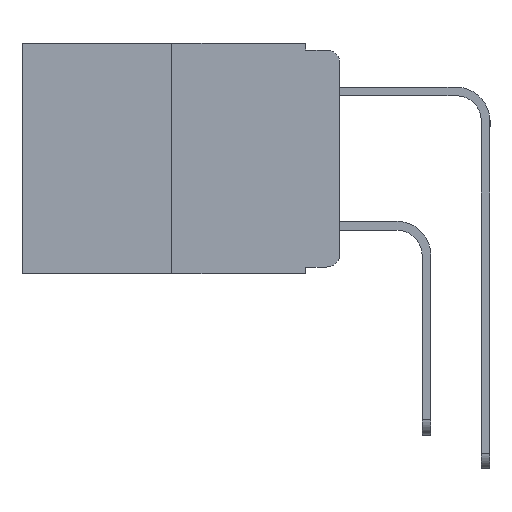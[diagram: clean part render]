
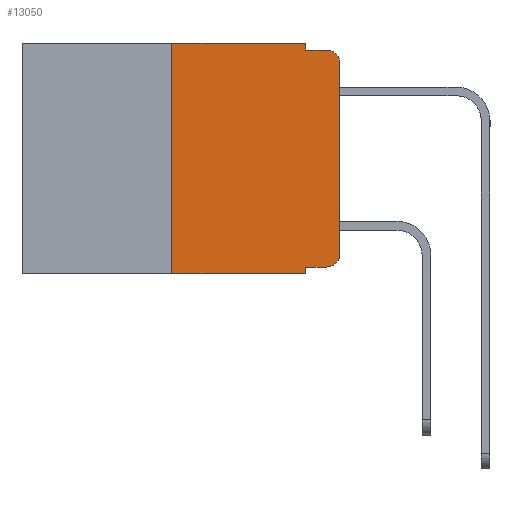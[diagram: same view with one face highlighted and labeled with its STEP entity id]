
A CAD part, left-side view. The second image highlights one B-rep face of the part: STEP entity #13050.
In plain terms, the highlighted planar face has unit normal (-1, 0, 0).
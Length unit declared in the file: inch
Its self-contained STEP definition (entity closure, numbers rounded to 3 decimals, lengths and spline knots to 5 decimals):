
#21 = CARTESIAN_POINT ( 'NONE',  ( 0., 0.051, -0.343 ) ) ;
#23 = CARTESIAN_POINT ( 'NONE',  ( 0., 0.02, -0.313 ) ) ;
#226 = EDGE_CURVE ( 'NONE', #5284, #3905, #3051, .T. ) ;
#235 = VECTOR ( 'NONE', #8747, 39.37008 ) ;
#519 = DIRECTION ( 'NONE',  ( 1., 0., 0. ) ) ;
#1103 = EDGE_CURVE ( 'NONE', #12461, #7772, #3863, .T. ) ;
#1113 = VERTEX_POINT ( 'NONE', #21 ) ;
#1264 = ORIENTED_EDGE ( 'NONE', *, *, #11909, .T. ) ;
#1349 = DIRECTION ( 'NONE',  ( 0., 0., -1. ) ) ;
#1474 = VERTEX_POINT ( 'NONE', #14182 ) ;
#1689 = ORIENTED_EDGE ( 'NONE', *, *, #14249, .F. ) ;
#1947 = EDGE_CURVE ( 'NONE', #7772, #6663, #12931, .T. ) ;
#2248 = CARTESIAN_POINT ( 'NONE',  ( 0., 0.051, 0. ) ) ;
#2265 = ORIENTED_EDGE ( 'NONE', *, *, #1947, .F. ) ;
#2275 = EDGE_LOOP ( 'NONE', ( #10076, #11959, #2265, #11504, #1689, #5946, #6763, #6268, #1264, #14040 ) ) ;
#2479 = CARTESIAN_POINT ( 'NONE',  ( 0., 0.473, -0.343 ) ) ;
#2789 = EDGE_CURVE ( 'NONE', #13586, #6663, #13840, .T. ) ;
#2926 = DIRECTION ( 'NONE',  ( -1., 0., 0. ) ) ;
#2942 = VERTEX_POINT ( 'NONE', #5293 ) ;
#2943 = VECTOR ( 'NONE', #12343, 39.37008 ) ;
#2957 = CARTESIAN_POINT ( 'NONE',  ( 0., 0.02, -0.03 ) ) ;
#3022 = CIRCLE ( 'NONE', #9111, 0.02 ) ;
#3051 = LINE ( 'NONE', #4029, #14140 ) ;
#3410 = CARTESIAN_POINT ( 'NONE',  ( 0., 0.02, -0.01 ) ) ;
#3563 = LINE ( 'NONE', #6613, #235 ) ;
#3581 = EDGE_CURVE ( 'NONE', #2942, #13586, #3563, .T. ) ;
#3640 = CARTESIAN_POINT ( 'NONE',  ( 0., 0.051, -0.333 ) ) ;
#3863 = LINE ( 'NONE', #4361, #6535 ) ;
#3905 = VERTEX_POINT ( 'NONE', #7463 ) ;
#4029 = CARTESIAN_POINT ( 'NONE',  ( 0., 0.25, 0. ) ) ;
#4361 = CARTESIAN_POINT ( 'NONE',  ( 0., 0.051, 0. ) ) ;
#5284 = VERTEX_POINT ( 'NONE', #13035 ) ;
#5293 = CARTESIAN_POINT ( 'NONE',  ( 0., 0., -0.313 ) ) ;
#5339 = PLANE ( 'NONE',  #6582 ) ;
#5773 = DIRECTION ( 'NONE',  ( 0., 0., 1. ) ) ;
#5905 = DIRECTION ( 'NONE',  ( 0., 0., -1. ) ) ;
#5946 = ORIENTED_EDGE ( 'NONE', *, *, #226, .F. ) ;
#6015 = LINE ( 'NONE', #2479, #2943 ) ;
#6268 = ORIENTED_EDGE ( 'NONE', *, *, #12588, .F. ) ;
#6535 = VECTOR ( 'NONE', #11933, 39.37008 ) ;
#6577 = LINE ( 'NONE', #2248, #12540 ) ;
#6582 = AXIS2_PLACEMENT_3D ( 'NONE', #7554, #519, #8621 ) ;
#6613 = CARTESIAN_POINT ( 'NONE',  ( 0., 0., 0. ) ) ;
#6663 = VERTEX_POINT ( 'NONE', #3410 ) ;
#6763 = ORIENTED_EDGE ( 'NONE', *, *, #14069, .T. ) ;
#7049 = DIRECTION ( 'NONE',  ( 0., -1., 0. ) ) ;
#7208 = LINE ( 'NONE', #11573, #9709 ) ;
#7332 = VERTEX_POINT ( 'NONE', #12303 ) ;
#7463 = CARTESIAN_POINT ( 'NONE',  ( 0., 0.25, 0. ) ) ;
#7554 = CARTESIAN_POINT ( 'NONE',  ( 0., 0.473, 0. ) ) ;
#7614 = VECTOR ( 'NONE', #7049, 39.37008 ) ;
#7768 = CARTESIAN_POINT ( 'NONE',  ( 0., 0.051, 0. ) ) ;
#7772 = VERTEX_POINT ( 'NONE', #9752 ) ;
#8255 = DIRECTION ( 'NONE',  ( -1., 0., 0. ) ) ;
#8497 = CARTESIAN_POINT ( 'NONE',  ( 0., 0., -0.03 ) ) ;
#8621 = DIRECTION ( 'NONE',  ( 0., 0., -1. ) ) ;
#8747 = DIRECTION ( 'NONE',  ( 0., 0., 1. ) ) ;
#9111 = AXIS2_PLACEMENT_3D ( 'NONE', #23, #8255, #1349 ) ;
#9172 = DIRECTION ( 'NONE',  ( 0., -1., 0. ) ) ;
#9709 = VECTOR ( 'NONE', #13568, 39.37008 ) ;
#9752 = CARTESIAN_POINT ( 'NONE',  ( 0., 0.051, -0.01 ) ) ;
#10076 = ORIENTED_EDGE ( 'NONE', *, *, #3581, .T. ) ;
#10086 = DIRECTION ( 'NONE',  ( 0., 0., -1. ) ) ;
#10180 = VECTOR ( 'NONE', #9172, 39.37008 ) ;
#10457 = LINE ( 'NONE', #3640, #7614 ) ;
#11097 = CARTESIAN_POINT ( 'NONE',  ( 0., 0.051, -0.01 ) ) ;
#11167 = AXIS2_PLACEMENT_3D ( 'NONE', #2957, #2926, #5905 ) ;
#11227 = EDGE_CURVE ( 'NONE', #1474, #2942, #3022, .T. ) ;
#11504 = ORIENTED_EDGE ( 'NONE', *, *, #1103, .F. ) ;
#11573 = CARTESIAN_POINT ( 'NONE',  ( 0., 0.473, 0. ) ) ;
#11909 = EDGE_CURVE ( 'NONE', #7332, #1474, #10457, .T. ) ;
#11933 = DIRECTION ( 'NONE',  ( 0., 0., -1. ) ) ;
#11959 = ORIENTED_EDGE ( 'NONE', *, *, #2789, .T. ) ;
#12303 = CARTESIAN_POINT ( 'NONE',  ( 0., 0.051, -0.333 ) ) ;
#12343 = DIRECTION ( 'NONE',  ( 0., -1., 0. ) ) ;
#12461 = VERTEX_POINT ( 'NONE', #7768 ) ;
#12540 = VECTOR ( 'NONE', #10086, 39.37008 ) ;
#12588 = EDGE_CURVE ( 'NONE', #7332, #1113, #6577, .T. ) ;
#12931 = LINE ( 'NONE', #11097, #10180 ) ;
#13035 = CARTESIAN_POINT ( 'NONE',  ( 0., 0.25, -0.343 ) ) ;
#13050 = ADVANCED_FACE ( 'NONE', ( #13139 ), #5339, .F. ) ;
#13139 = FACE_OUTER_BOUND ( 'NONE', #2275, .T. ) ;
#13568 = DIRECTION ( 'NONE',  ( 0., -1., 0. ) ) ;
#13586 = VERTEX_POINT ( 'NONE', #8497 ) ;
#13840 = CIRCLE ( 'NONE', #11167, 0.02 ) ;
#14040 = ORIENTED_EDGE ( 'NONE', *, *, #11227, .T. ) ;
#14069 = EDGE_CURVE ( 'NONE', #5284, #1113, #6015, .T. ) ;
#14140 = VECTOR ( 'NONE', #5773, 39.37008 ) ;
#14182 = CARTESIAN_POINT ( 'NONE',  ( 0., 0.02, -0.333 ) ) ;
#14249 = EDGE_CURVE ( 'NONE', #3905, #12461, #7208, .T. ) ;
